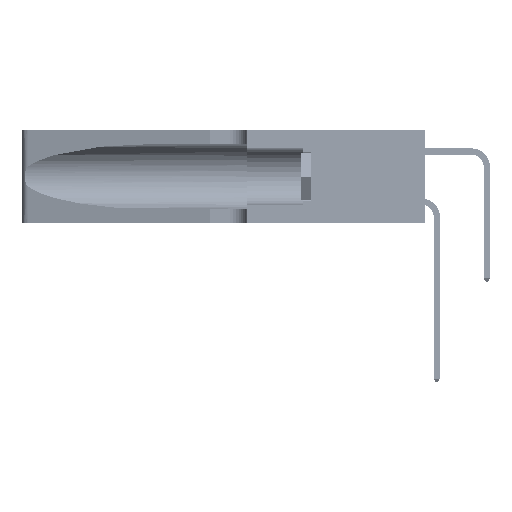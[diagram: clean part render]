
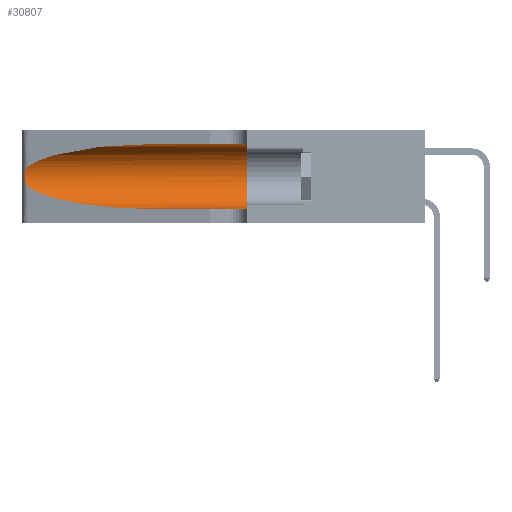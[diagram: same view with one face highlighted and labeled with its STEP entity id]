
A CAD part, left-side view. The second image highlights one B-rep face of the part: STEP entity #30807.
In plain terms, the highlighted cylindrical face has radius 3.308 mm (diameter 6.617 mm), a partial arc.
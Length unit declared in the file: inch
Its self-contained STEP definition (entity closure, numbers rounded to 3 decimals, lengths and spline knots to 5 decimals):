
#181 = CARTESIAN_POINT ( 'NONE',  ( 0.1305, 0.35, 0.05475 ) ) ;
#2848 = CARTESIAN_POINT ( 'NONE',  ( 0.25789, 1.23486, 0.15765 ) ) ;
#4623 = EDGE_CURVE ( 'NONE', #18434, #41829, #25872, .T. ) ;
#4914 = ORIENTED_EDGE ( 'NONE', *, *, #17877, .T. ) ;
#4994 = ORIENTED_EDGE ( 'NONE', *, *, #6866, .T. ) ;
#6479 = CARTESIAN_POINT ( 'NONE',  ( 0.25487, 1.22718, 0.22369 ) ) ;
#6490 = CARTESIAN_POINT ( 'NONE',  ( 0.1305, 0.72297, 0.05475 ) ) ;
#6645 = CARTESIAN_POINT ( 'NONE',  ( 0.25555, 1.22994, 0.2215 ) ) ;
#6819 = CARTESIAN_POINT ( 'NONE',  ( 0.25555, 1.22993, 0.14849 ) ) ;
#6866 = EDGE_CURVE ( 'NONE', #37135, #28407, #12302, .T. ) ;
#8057 = EDGE_CURVE ( 'NONE', #25586, #8877, #45320, .T. ) ;
#8560 = VECTOR ( 'NONE', #49135, 39.37008 ) ;
#8877 = VERTEX_POINT ( 'NONE', #44925 ) ;
#9685 = CARTESIAN_POINT ( 'NONE',  ( 0.1305, 1.61858, 0.185 ) ) ;
#10715 = CARTESIAN_POINT ( 'NONE',  ( 0.25487, 1.22718, 0.14631 ) ) ;
#10753 = CARTESIAN_POINT ( 'NONE',  ( 0.1305, 0.72297, 0.31525 ) ) ;
#12178 =( BOUNDED_CURVE ( )  B_SPLINE_CURVE ( 3, ( #25461, #45094, #41314, #17688 ),
 .UNSPECIFIED., .F., .F. ) 
 B_SPLINE_CURVE_WITH_KNOTS ( ( 4, 4 ),
 ( 3.44316, 4.71239 ),
 .UNSPECIFIED. ) 
 CURVE ( )  GEOMETRIC_REPRESENTATION_ITEM ( )  RATIONAL_B_SPLINE_CURVE ( ( 1., 0.87, 0.87, 1. ) ) 
 REPRESENTATION_ITEM ( '' )  );
#12302 = B_SPLINE_CURVE_WITH_KNOTS ( 'NONE', 3,
 ( #38256, #6645, #49947, #14659, #42224, #18626, #46157, #22571, #50115, #26542, #2848, #30527, #6819, #34477 ),
 .UNSPECIFIED., .F., .F.,
 ( 4, 2, 2, 2, 2, 2, 4 ),
 ( 0., 0.00027, 0.00053, 0.00107, 0.0016, 0.00187, 0.00214 ),
 .UNSPECIFIED. ) ;
#13109 = ORIENTED_EDGE ( 'NONE', *, *, #8057, .F. ) ;
#13272 = ORIENTED_EDGE ( 'NONE', *, *, #4623, .T. ) ;
#14025 = CARTESIAN_POINT ( 'NONE',  ( 0.25487, 1.22718, 0.22369 ) ) ;
#14366 = CARTESIAN_POINT ( 'NONE',  ( 0.1305, 1.61858, 0.31525 ) ) ;
#14659 = CARTESIAN_POINT ( 'NONE',  ( 0.25787, 1.23484, 0.2124 ) ) ;
#17607 = CARTESIAN_POINT ( 'NONE',  ( 0.1305, 1.61858, 0.05475 ) ) ;
#17688 = CARTESIAN_POINT ( 'NONE',  ( 0.1305, 0.72297, 0.05475 ) ) ;
#17877 = EDGE_CURVE ( 'NONE', #28407, #18434, #12178, .T. ) ;
#18434 = VERTEX_POINT ( 'NONE', #6490 ) ;
#18626 = CARTESIAN_POINT ( 'NONE',  ( 0.26018, 1.23835, 0.19895 ) ) ;
#20742 = DIRECTION ( 'NONE',  ( 0., 1., 0. ) ) ;
#22571 = CARTESIAN_POINT ( 'NONE',  ( 0.26075, 1.23896, 0.178 ) ) ;
#23127 = AXIS2_PLACEMENT_3D ( 'NONE', #44360, #20742, #48285 ) ;
#25461 = CARTESIAN_POINT ( 'NONE',  ( 0.25487, 1.22718, 0.14631 ) ) ;
#25586 = VERTEX_POINT ( 'NONE', #10753 ) ;
#25872 = LINE ( 'NONE', #17607, #8560 ) ;
#26210 = CARTESIAN_POINT ( 'NONE',  ( 0.1305, 0.72297, 0.31525 ) ) ;
#26542 = CARTESIAN_POINT ( 'NONE',  ( 0.25856, 1.23593, 0.16098 ) ) ;
#26603 = CYLINDRICAL_SURFACE ( 'NONE', #30478, 0.13025 ) ;
#26763 = EDGE_LOOP ( 'NONE', ( #43819, #4994, #4914, #13272, #37992, #13109 ) ) ;
#28407 = VERTEX_POINT ( 'NONE', #10715 ) ;
#28612 = EDGE_CURVE ( 'NONE', #8877, #41829, #43387, .T. ) ;
#30187 = CARTESIAN_POINT ( 'NONE',  ( 0.2373, 1.15595, 0.28018 ) ) ;
#30478 = AXIS2_PLACEMENT_3D ( 'NONE', #9685, #41100, #33350 ) ;
#30527 = CARTESIAN_POINT ( 'NONE',  ( 0.25639, 1.23186, 0.15144 ) ) ;
#30807 = ADVANCED_FACE ( 'NONE', ( #47522 ), #26603, .F. ) ;
#31580 = EDGE_CURVE ( 'NONE', #25586, #37135, #48884, .T. ) ;
#33350 = DIRECTION ( 'NONE',  ( 0., 0., -1. ) ) ;
#34477 = CARTESIAN_POINT ( 'NONE',  ( 0.25487, 1.22718, 0.14631 ) ) ;
#37135 = VERTEX_POINT ( 'NONE', #14025 ) ;
#37977 = DIRECTION ( 'NONE',  ( 0., -1., 0. ) ) ;
#37992 = ORIENTED_EDGE ( 'NONE', *, *, #28612, .F. ) ;
#38256 = CARTESIAN_POINT ( 'NONE',  ( 0.25487, 1.22718, 0.22369 ) ) ;
#41100 = DIRECTION ( 'NONE',  ( 0., -1., 0. ) ) ;
#41314 = CARTESIAN_POINT ( 'NONE',  ( 0.18966, 0.96281, 0.05475 ) ) ;
#41829 = VERTEX_POINT ( 'NONE', #181 ) ;
#42224 = CARTESIAN_POINT ( 'NONE',  ( 0.25854, 1.2359, 0.20912 ) ) ;
#43387 = CIRCLE ( 'NONE', #23127, 0.13025 ) ;
#43819 = ORIENTED_EDGE ( 'NONE', *, *, #31580, .T. ) ;
#44096 = VECTOR ( 'NONE', #37977, 39.37008 ) ;
#44360 = CARTESIAN_POINT ( 'NONE',  ( 0.1305, 0.35, 0.185 ) ) ;
#44925 = CARTESIAN_POINT ( 'NONE',  ( 0.1305, 0.35, 0.31525 ) ) ;
#45094 = CARTESIAN_POINT ( 'NONE',  ( 0.2373, 1.15595, 0.08982 ) ) ;
#45320 = LINE ( 'NONE', #14366, #44096 ) ;
#45825 = CARTESIAN_POINT ( 'NONE',  ( 0.18966, 0.96281, 0.31525 ) ) ;
#46157 = CARTESIAN_POINT ( 'NONE',  ( 0.26075, 1.23896, 0.19203 ) ) ;
#47522 = FACE_OUTER_BOUND ( 'NONE', #26763, .T. ) ;
#48285 = DIRECTION ( 'NONE',  ( 0., 0., 1. ) ) ;
#48884 =( BOUNDED_CURVE ( )  B_SPLINE_CURVE ( 3, ( #26210, #45825, #30187, #6479 ),
 .UNSPECIFIED., .F., .T. ) 
 B_SPLINE_CURVE_WITH_KNOTS ( ( 4, 4 ),
 ( 1.5708, 2.84003 ),
 .UNSPECIFIED. ) 
 CURVE ( )  GEOMETRIC_REPRESENTATION_ITEM ( )  RATIONAL_B_SPLINE_CURVE ( ( 1., 0.87, 0.87, 1. ) ) 
 REPRESENTATION_ITEM ( '' )  );
#49135 = DIRECTION ( 'NONE',  ( 0., -1., 0. ) ) ;
#49947 = CARTESIAN_POINT ( 'NONE',  ( 0.25639, 1.23184, 0.21858 ) ) ;
#50115 = CARTESIAN_POINT ( 'NONE',  ( 0.26017, 1.23833, 0.17102 ) ) ;
